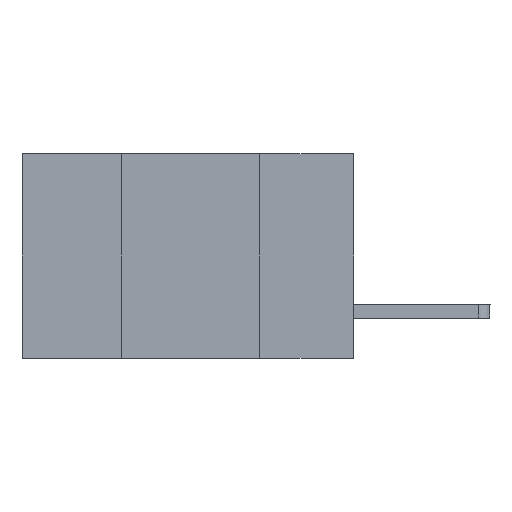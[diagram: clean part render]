
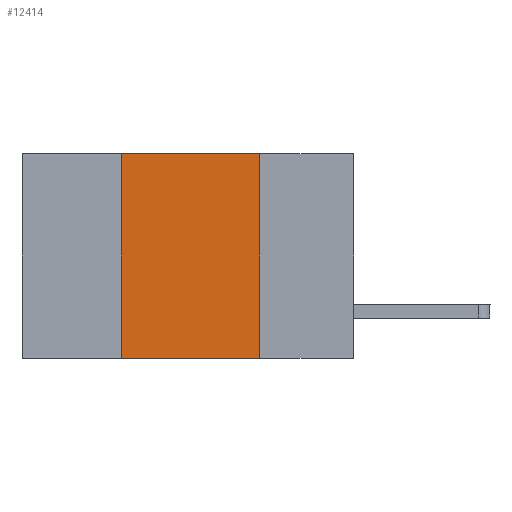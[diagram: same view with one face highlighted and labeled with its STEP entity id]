
A CAD part, left-side view. The second image highlights one B-rep face of the part: STEP entity #12414.
In plain terms, the highlighted planar face has unit normal (-1, 0, 0).
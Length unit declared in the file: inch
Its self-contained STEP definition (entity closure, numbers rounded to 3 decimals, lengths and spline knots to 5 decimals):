
#285 = CARTESIAN_POINT ( 'NONE',  ( 0., 0.42, -0.37 ) ) ;
#713 = VECTOR ( 'NONE', #7925, 39.37008 ) ;
#715 = ORIENTED_EDGE ( 'NONE', *, *, #10831, .F. ) ;
#729 = DIRECTION ( 'NONE',  ( 0., -1., 0. ) ) ;
#761 = CARTESIAN_POINT ( 'NONE',  ( 0., 0.6, -0.37 ) ) ;
#864 = VECTOR ( 'NONE', #2715, 39.37008 ) ;
#1264 = VERTEX_POINT ( 'NONE', #10817 ) ;
#1935 = EDGE_CURVE ( 'NONE', #9029, #4934, #6702, .T. ) ;
#2715 = DIRECTION ( 'NONE',  ( 0., 0., 1. ) ) ;
#2865 = DIRECTION ( 'NONE',  ( 0., 0., -1. ) ) ;
#3005 = CARTESIAN_POINT ( 'NONE',  ( 0., 0.42, 0. ) ) ;
#3572 = EDGE_CURVE ( 'NONE', #9029, #1264, #9835, .T. ) ;
#3577 = CARTESIAN_POINT ( 'NONE',  ( 0., 0.6, 0. ) ) ;
#4379 = CARTESIAN_POINT ( 'NONE',  ( 0., 0.42, 0. ) ) ;
#4754 = PLANE ( 'NONE',  #8406 ) ;
#4934 = VERTEX_POINT ( 'NONE', #3005 ) ;
#6250 = VECTOR ( 'NONE', #729, 39.37008 ) ;
#6324 = CARTESIAN_POINT ( 'NONE',  ( 0., 0.17, 0. ) ) ;
#6702 = LINE ( 'NONE', #4379, #864 ) ;
#6910 = EDGE_LOOP ( 'NONE', ( #7716, #715, #11028, #10687 ) ) ;
#7716 = ORIENTED_EDGE ( 'NONE', *, *, #10660, .F. ) ;
#7925 = DIRECTION ( 'NONE',  ( 0., 0., -1. ) ) ;
#8406 = AXIS2_PLACEMENT_3D ( 'NONE', #8497, #8573, #2865 ) ;
#8497 = CARTESIAN_POINT ( 'NONE',  ( 0., 0.6, 0. ) ) ;
#8573 = DIRECTION ( 'NONE',  ( 1., 0., 0. ) ) ;
#8629 = FACE_OUTER_BOUND ( 'NONE', #6910, .T. ) ;
#9029 = VERTEX_POINT ( 'NONE', #285 ) ;
#9835 = LINE ( 'NONE', #761, #10732 ) ;
#10364 = LINE ( 'NONE', #10963, #713 ) ;
#10413 = DIRECTION ( 'NONE',  ( 0., -1., 0. ) ) ;
#10660 = EDGE_CURVE ( 'NONE', #11425, #1264, #10364, .T. ) ;
#10687 = ORIENTED_EDGE ( 'NONE', *, *, #3572, .T. ) ;
#10732 = VECTOR ( 'NONE', #10413, 39.37008 ) ;
#10817 = CARTESIAN_POINT ( 'NONE',  ( 0., 0.17, -0.37 ) ) ;
#10831 = EDGE_CURVE ( 'NONE', #4934, #11425, #11565, .T. ) ;
#10963 = CARTESIAN_POINT ( 'NONE',  ( 0., 0.17, 0. ) ) ;
#11028 = ORIENTED_EDGE ( 'NONE', *, *, #1935, .F. ) ;
#11425 = VERTEX_POINT ( 'NONE', #6324 ) ;
#11565 = LINE ( 'NONE', #3577, #6250 ) ;
#12414 = ADVANCED_FACE ( 'NONE', ( #8629 ), #4754, .F. ) ;
